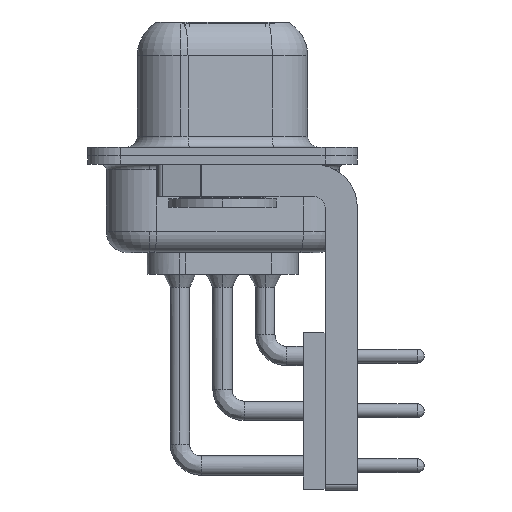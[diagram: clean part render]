
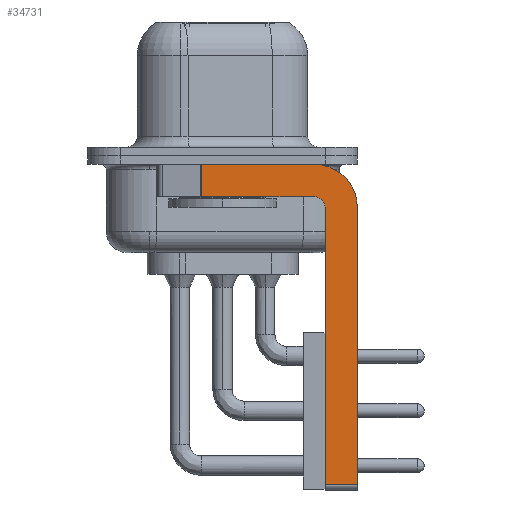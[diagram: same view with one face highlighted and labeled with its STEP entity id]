
A CAD part, left-side view. The second image highlights one B-rep face of the part: STEP entity #34731.
In plain terms, the highlighted planar face has unit normal (-1, 0, 0).
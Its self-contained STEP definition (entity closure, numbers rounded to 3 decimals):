
#1423 = EDGE_CURVE ( 'NONE', #18083, #3713, #19421, .T. ) ;
#3713 = VERTEX_POINT ( 'NONE', #15202 ) ;
#6237 = VERTEX_POINT ( 'NONE', #18483 ) ;
#6939 = CARTESIAN_POINT ( 'NONE',  ( -2.9, -6.25, -15.25 ) ) ;
#7087 = CARTESIAN_POINT ( 'NONE',  ( -2.9, -4.25, -15.25 ) ) ;
#7125 = CARTESIAN_POINT ( 'NONE',  ( -2.9, -4.25, -0.4 ) ) ;
#8056 = DIRECTION ( 'NONE',  ( 0., 0., -1. ) ) ;
#8112 = DIRECTION ( 'NONE',  ( 0., -1., 0. ) ) ;
#8701 = CARTESIAN_POINT ( 'NONE',  ( -2.9, -4.25, -1.9 ) ) ;
#8825 = VERTEX_POINT ( 'NONE', #33936 ) ;
#11246 = ORIENTED_EDGE ( 'NONE', *, *, #1423, .T. ) ;
#11414 = CARTESIAN_POINT ( 'NONE',  ( -2.9, -6.25, -2.4 ) ) ;
#11614 = CARTESIAN_POINT ( 'NONE',  ( -2.9, 0.978, -1.9 ) ) ;
#11827 = CARTESIAN_POINT ( 'NONE',  ( -2.9, -4.75, -15.5 ) ) ;
#11923 = CARTESIAN_POINT ( 'NONE',  ( -2.9, -4.25, -2.4 ) ) ;
#12016 = DIRECTION ( 'NONE',  ( 1., 0., 0. ) ) ;
#12850 = ORIENTED_EDGE ( 'NONE', *, *, #23996, .F. ) ;
#13036 = CARTESIAN_POINT ( 'NONE',  ( -2.9, -4.25, -2.4 ) ) ;
#13319 = CARTESIAN_POINT ( 'NONE',  ( -2.9, 0.978, -0.4 ) ) ;
#14012 = EDGE_CURVE ( 'NONE', #8825, #28548, #14738, .T. ) ;
#14248 = DIRECTION ( 'NONE',  ( 0., 1., 0. ) ) ;
#14696 = DIRECTION ( 'NONE',  ( 0., 0., -1. ) ) ;
#14738 = LINE ( 'NONE', #7087, #22777 ) ;
#14861 = FACE_OUTER_BOUND ( 'NONE', #26034, .T. ) ;
#15202 = CARTESIAN_POINT ( 'NONE',  ( -2.9, 0.978, -1.9 ) ) ;
#15816 = DIRECTION ( 'NONE',  ( 0., 0., 1. ) ) ;
#16095 = VECTOR ( 'NONE', #14248, 1000. ) ;
#16368 = CARTESIAN_POINT ( 'NONE',  ( -2.9, 3., -0.4 ) ) ;
#16708 = ORIENTED_EDGE ( 'NONE', *, *, #19012, .F. ) ;
#18083 = VERTEX_POINT ( 'NONE', #13319 ) ;
#18317 = VECTOR ( 'NONE', #28113, 1000. ) ;
#18483 = CARTESIAN_POINT ( 'NONE',  ( -2.9, -4.25, -1.9 ) ) ;
#18778 = CARTESIAN_POINT ( 'NONE',  ( -2.9, -6.25, -2.4 ) ) ;
#19012 = EDGE_CURVE ( 'NONE', #8825, #25452, #24692, .T. ) ;
#19391 = AXIS2_PLACEMENT_3D ( 'NONE', #13036, #32068, #15816 ) ;
#19421 = LINE ( 'NONE', #11614, #24096 ) ;
#19554 = EDGE_CURVE ( 'NONE', #21915, #26043, #32773, .T. ) ;
#20177 = VECTOR ( 'NONE', #8056, 1000. ) ;
#20219 = CARTESIAN_POINT ( 'NONE',  ( -2.9, -4.25, -2.4 ) ) ;
#20344 = LINE ( 'NONE', #16368, #34031 ) ;
#20484 = EDGE_CURVE ( 'NONE', #18083, #21915, #20344, .T. ) ;
#20597 = EDGE_CURVE ( 'NONE', #6237, #3713, #24995, .T. ) ;
#21364 = CIRCLE ( 'NONE', #19391, 0.5 ) ;
#21915 = VERTEX_POINT ( 'NONE', #7125 ) ;
#22024 = DIRECTION ( 'NONE',  ( 0., 0., -1. ) ) ;
#22777 = VECTOR ( 'NONE', #23433, 1000. ) ;
#22953 = AXIS2_PLACEMENT_3D ( 'NONE', #20219, #12016, #25702 ) ;
#22963 = PLANE ( 'NONE',  #22953 ) ;
#23433 = DIRECTION ( 'NONE',  ( 0., -1., 0. ) ) ;
#23996 = EDGE_CURVE ( 'NONE', #26043, #28548, #27401, .T. ) ;
#24096 = VECTOR ( 'NONE', #22024, 1000. ) ;
#24692 = LINE ( 'NONE', #11827, #18317 ) ;
#24995 = LINE ( 'NONE', #8701, #16095 ) ;
#25452 = VERTEX_POINT ( 'NONE', #33274 ) ;
#25702 = DIRECTION ( 'NONE',  ( 0., 0., -1. ) ) ;
#25895 = ORIENTED_EDGE ( 'NONE', *, *, #19554, .F. ) ;
#26034 = EDGE_LOOP ( 'NONE', ( #31480, #11246, #32566, #33115, #16708, #35040, #12850, #25895 ) ) ;
#26043 = VERTEX_POINT ( 'NONE', #11414 ) ;
#27401 = LINE ( 'NONE', #18778, #20177 ) ;
#28113 = DIRECTION ( 'NONE',  ( 0., 0., 1. ) ) ;
#28548 = VERTEX_POINT ( 'NONE', #6939 ) ;
#30924 = EDGE_CURVE ( 'NONE', #25452, #6237, #21364, .T. ) ;
#30941 = DIRECTION ( 'NONE',  ( 1., 0., 0. ) ) ;
#31480 = ORIENTED_EDGE ( 'NONE', *, *, #20484, .F. ) ;
#32068 = DIRECTION ( 'NONE',  ( -1., 0., 0. ) ) ;
#32566 = ORIENTED_EDGE ( 'NONE', *, *, #20597, .F. ) ;
#32773 = CIRCLE ( 'NONE', #34014, 2. ) ;
#33115 = ORIENTED_EDGE ( 'NONE', *, *, #30924, .F. ) ;
#33274 = CARTESIAN_POINT ( 'NONE',  ( -2.9, -4.75, -2.4 ) ) ;
#33936 = CARTESIAN_POINT ( 'NONE',  ( -2.9, -4.75, -15.25 ) ) ;
#34014 = AXIS2_PLACEMENT_3D ( 'NONE', #11923, #30941, #14696 ) ;
#34031 = VECTOR ( 'NONE', #8112, 1000. ) ;
#34731 = ADVANCED_FACE ( 'NONE', ( #14861 ), #22963, .F. ) ;
#35040 = ORIENTED_EDGE ( 'NONE', *, *, #14012, .T. ) ;
